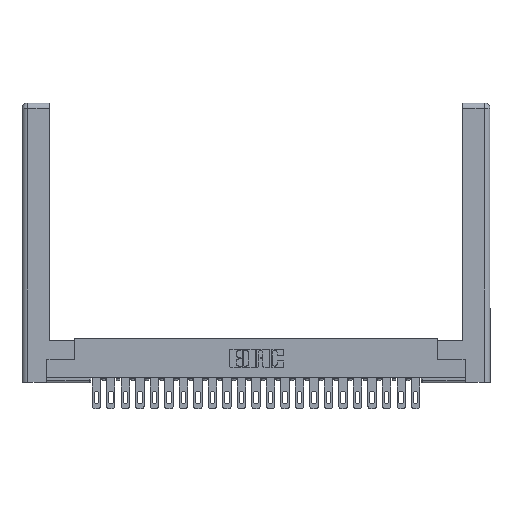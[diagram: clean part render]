
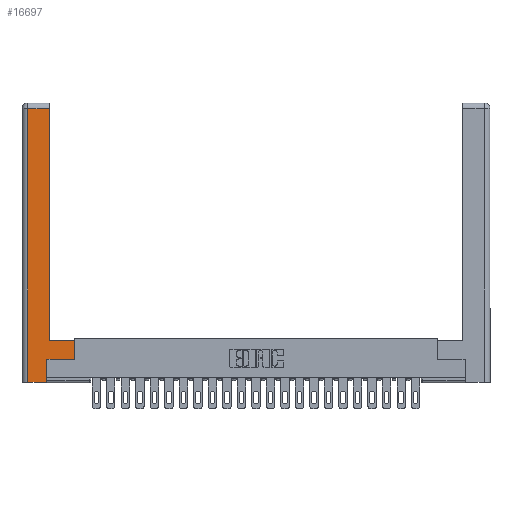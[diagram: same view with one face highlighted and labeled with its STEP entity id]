
A CAD part, top view. The second image highlights one B-rep face of the part: STEP entity #16697.
In plain terms, the highlighted planar face has unit normal (0, 0, 1).
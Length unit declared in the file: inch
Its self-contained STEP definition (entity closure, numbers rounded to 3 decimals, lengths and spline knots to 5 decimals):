
#757 = AXIS2_PLACEMENT_3D ( 'NONE', #24493, #20771, #21147 ) ;
#877 = LINE ( 'NONE', #20124, #16114 ) ;
#897 = CARTESIAN_POINT ( 'NONE',  ( 0.0615, 0., 0. ) ) ;
#1313 = EDGE_CURVE ( 'NONE', #9218, #21655, #10421, .T. ) ;
#1634 = LINE ( 'NONE', #21009, #23843 ) ;
#2085 = ORIENTED_EDGE ( 'NONE', *, *, #8176, .T. ) ;
#2149 = ORIENTED_EDGE ( 'NONE', *, *, #1313, .T. ) ;
#2436 = LINE ( 'NONE', #23422, #11368 ) ;
#2888 = ORIENTED_EDGE ( 'NONE', *, *, #15585, .T. ) ;
#2911 = VERTEX_POINT ( 'NONE', #897 ) ;
#3320 = VECTOR ( 'NONE', #10165, 39.37008 ) ;
#3733 = DIRECTION ( 'NONE',  ( 0., 1., 0. ) ) ;
#4308 = CARTESIAN_POINT ( 'NONE',  ( 0.295, 2.94, 0. ) ) ;
#4681 = DIRECTION ( 'NONE',  ( -1., 0., 0. ) ) ;
#5349 = VECTOR ( 'NONE', #7966, 39.37008 ) ;
#5427 = CARTESIAN_POINT ( 'NONE',  ( 0.265, 0.245, 0. ) ) ;
#6482 = ORIENTED_EDGE ( 'NONE', *, *, #18079, .T. ) ;
#6512 = CARTESIAN_POINT ( 'NONE',  ( 0.265, 0.245, 0. ) ) ;
#6799 = LINE ( 'NONE', #18166, #16903 ) ;
#6827 = EDGE_CURVE ( 'NONE', #15082, #23792, #23418, .T. ) ;
#7966 = DIRECTION ( 'NONE',  ( 0., -1., 0. ) ) ;
#8176 = EDGE_CURVE ( 'NONE', #10771, #2911, #9718, .T. ) ;
#8330 = FACE_OUTER_BOUND ( 'NONE', #17777, .T. ) ;
#9218 = VERTEX_POINT ( 'NONE', #23851 ) ;
#9718 = LINE ( 'NONE', #19215, #5349 ) ;
#9987 = ORIENTED_EDGE ( 'NONE', *, *, #20431, .T. ) ;
#10165 = DIRECTION ( 'NONE',  ( -1., 0., 0. ) ) ;
#10421 = LINE ( 'NONE', #19661, #3320 ) ;
#10771 = VERTEX_POINT ( 'NONE', #20625 ) ;
#10779 = DIRECTION ( 'NONE',  ( 0., 1., 0. ) ) ;
#10824 = CARTESIAN_POINT ( 'NONE',  ( 0.565, 0.245, 0. ) ) ;
#10894 = VERTEX_POINT ( 'NONE', #23109 ) ;
#10962 = ORIENTED_EDGE ( 'NONE', *, *, #22479, .T. ) ;
#11368 = VECTOR ( 'NONE', #4681, 39.37008 ) ;
#11956 = CARTESIAN_POINT ( 'NONE',  ( 0.565, 0.245, 0. ) ) ;
#14481 = DIRECTION ( 'NONE',  ( 1., 0., 0. ) ) ;
#14928 = DIRECTION ( 'NONE',  ( 0., 1., 0. ) ) ;
#15082 = VERTEX_POINT ( 'NONE', #6512 ) ;
#15585 = EDGE_CURVE ( 'NONE', #23792, #9218, #1634, .T. ) ;
#15957 = ORIENTED_EDGE ( 'NONE', *, *, #21747, .T. ) ;
#16114 = VECTOR ( 'NONE', #14481, 39.37008 ) ;
#16293 = PLANE ( 'NONE',  #757 ) ;
#16697 = ADVANCED_FACE ( 'NONE', ( #8330 ), #16293, .F. ) ;
#16903 = VECTOR ( 'NONE', #10779, 39.37008 ) ;
#17755 = VERTEX_POINT ( 'NONE', #4308 ) ;
#17777 = EDGE_LOOP ( 'NONE', ( #15957, #10962, #2085, #9987, #6482, #21076, #2888, #2149 ) ) ;
#18079 = EDGE_CURVE ( 'NONE', #10894, #15082, #22672, .T. ) ;
#18166 = CARTESIAN_POINT ( 'NONE',  ( 0.295, 3., 0. ) ) ;
#19164 = VECTOR ( 'NONE', #14928, 39.37008 ) ;
#19215 = CARTESIAN_POINT ( 'NONE',  ( 0.0615, 0., 0. ) ) ;
#19476 = VECTOR ( 'NONE', #19576, 39.37008 ) ;
#19576 = DIRECTION ( 'NONE',  ( 1., 0., 0. ) ) ;
#19657 = CARTESIAN_POINT ( 'NONE',  ( 0.295, 0.45, 0. ) ) ;
#19661 = CARTESIAN_POINT ( 'NONE',  ( 0.295, 0.45, 0. ) ) ;
#20124 = CARTESIAN_POINT ( 'NONE',  ( 0.265, 0., 0. ) ) ;
#20431 = EDGE_CURVE ( 'NONE', #2911, #10894, #877, .T. ) ;
#20625 = CARTESIAN_POINT ( 'NONE',  ( 0.0615, 2.94, 0. ) ) ;
#20771 = DIRECTION ( 'NONE',  ( 0., 0., -1. ) ) ;
#21009 = CARTESIAN_POINT ( 'NONE',  ( 0.565, 0.45, 0. ) ) ;
#21076 = ORIENTED_EDGE ( 'NONE', *, *, #6827, .T. ) ;
#21147 = DIRECTION ( 'NONE',  ( -1., 0., 0. ) ) ;
#21655 = VERTEX_POINT ( 'NONE', #19657 ) ;
#21747 = EDGE_CURVE ( 'NONE', #21655, #17755, #6799, .T. ) ;
#22479 = EDGE_CURVE ( 'NONE', #17755, #10771, #2436, .T. ) ;
#22672 = LINE ( 'NONE', #5427, #19164 ) ;
#23109 = CARTESIAN_POINT ( 'NONE',  ( 0.265, 0., 0. ) ) ;
#23418 = LINE ( 'NONE', #11956, #19476 ) ;
#23422 = CARTESIAN_POINT ( 'NONE',  ( 0.0615, 2.94, 0. ) ) ;
#23792 = VERTEX_POINT ( 'NONE', #10824 ) ;
#23843 = VECTOR ( 'NONE', #3733, 39.37008 ) ;
#23851 = CARTESIAN_POINT ( 'NONE',  ( 0.565, 0.45, 0. ) ) ;
#24493 = CARTESIAN_POINT ( 'NONE',  ( 0., 0., 0. ) ) ;
